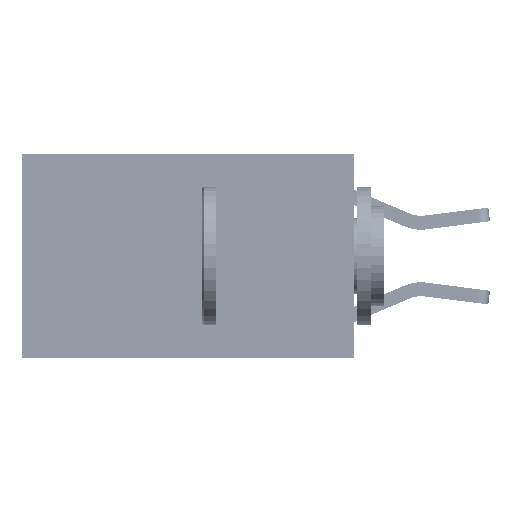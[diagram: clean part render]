
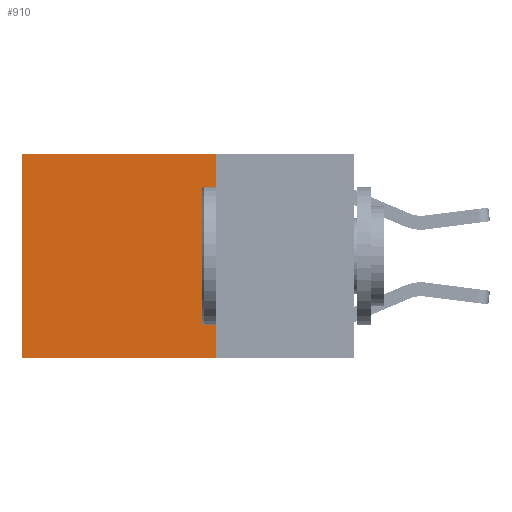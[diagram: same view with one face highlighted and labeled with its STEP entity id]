
A CAD part, left-side view. The second image highlights one B-rep face of the part: STEP entity #910.
In plain terms, the highlighted planar face has unit normal (-1, 0, 0).
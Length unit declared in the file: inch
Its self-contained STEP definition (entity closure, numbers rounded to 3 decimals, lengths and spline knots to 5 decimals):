
#232 = DIRECTION ( 'NONE',  ( 1., 0., 0. ) ) ;
#910 = ADVANCED_FACE ( 'NONE', ( #5325 ), #5652, .F. ) ;
#962 = VERTEX_POINT ( 'NONE', #25536 ) ;
#1422 = DIRECTION ( 'NONE',  ( 0., 1., 0. ) ) ;
#1690 = DIRECTION ( 'NONE',  ( 0., 0., -1. ) ) ;
#3732 = LINE ( 'NONE', #11772, #4288 ) ;
#4288 = VECTOR ( 'NONE', #1422, 39.37008 ) ;
#5325 = FACE_OUTER_BOUND ( 'NONE', #20476, .T. ) ;
#5652 = PLANE ( 'NONE',  #29739 ) ;
#7791 = EDGE_CURVE ( 'NONE', #8514, #11681, #19458, .T. ) ;
#8514 = VERTEX_POINT ( 'NONE', #19867 ) ;
#8685 = CARTESIAN_POINT ( 'NONE',  ( 0.2625, 0.25, 0. ) ) ;
#9594 = VECTOR ( 'NONE', #19965, 39.37008 ) ;
#11559 = EDGE_CURVE ( 'NONE', #12755, #8514, #3732, .T. ) ;
#11681 = VERTEX_POINT ( 'NONE', #24911 ) ;
#11772 = CARTESIAN_POINT ( 'NONE',  ( 0.2625, 0.25, 0. ) ) ;
#12227 = LINE ( 'NONE', #29649, #9594 ) ;
#12386 = LINE ( 'NONE', #22408, #19514 ) ;
#12755 = VERTEX_POINT ( 'NONE', #8685 ) ;
#15151 = VECTOR ( 'NONE', #1690, 39.37008 ) ;
#15485 = ORIENTED_EDGE ( 'NONE', *, *, #25840, .F. ) ;
#17662 = DIRECTION ( 'NONE',  ( 0., 0., -1. ) ) ;
#19458 = LINE ( 'NONE', #26692, #15151 ) ;
#19514 = VECTOR ( 'NONE', #29972, 39.37008 ) ;
#19867 = CARTESIAN_POINT ( 'NONE',  ( 0.2625, 0.6, 0. ) ) ;
#19965 = DIRECTION ( 'NONE',  ( 0., 1., 0. ) ) ;
#20476 = EDGE_LOOP ( 'NONE', ( #26933, #15485, #21306, #25800 ) ) ;
#21306 = ORIENTED_EDGE ( 'NONE', *, *, #24231, .F. ) ;
#22408 = CARTESIAN_POINT ( 'NONE',  ( 0.2625, 0.25, 0. ) ) ;
#22735 = CARTESIAN_POINT ( 'NONE',  ( 0.2625, 0.25, 0. ) ) ;
#24231 = EDGE_CURVE ( 'NONE', #12755, #962, #12386, .T. ) ;
#24911 = CARTESIAN_POINT ( 'NONE',  ( 0.2625, 0.6, -0.37 ) ) ;
#25536 = CARTESIAN_POINT ( 'NONE',  ( 0.2625, 0.25, -0.37 ) ) ;
#25800 = ORIENTED_EDGE ( 'NONE', *, *, #11559, .T. ) ;
#25840 = EDGE_CURVE ( 'NONE', #962, #11681, #12227, .T. ) ;
#26692 = CARTESIAN_POINT ( 'NONE',  ( 0.2625, 0.6, 0. ) ) ;
#26933 = ORIENTED_EDGE ( 'NONE', *, *, #7791, .T. ) ;
#29649 = CARTESIAN_POINT ( 'NONE',  ( 0.2625, 0.25, -0.37 ) ) ;
#29739 = AXIS2_PLACEMENT_3D ( 'NONE', #22735, #232, #17662 ) ;
#29972 = DIRECTION ( 'NONE',  ( 0., 0., -1. ) ) ;
